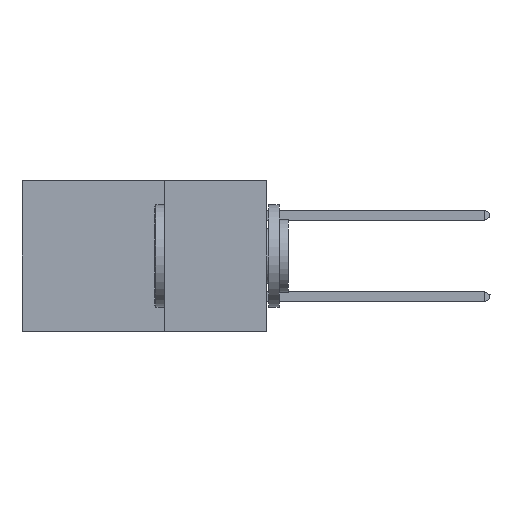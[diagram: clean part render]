
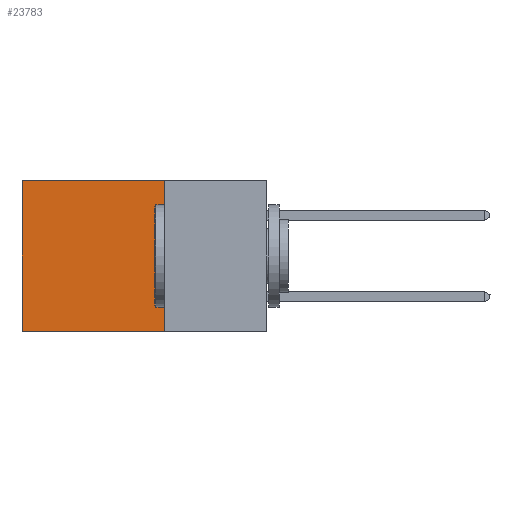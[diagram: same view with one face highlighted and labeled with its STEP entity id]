
A CAD part, left-side view. The second image highlights one B-rep face of the part: STEP entity #23783.
In plain terms, the highlighted planar face has unit normal (-1, 0, 0).
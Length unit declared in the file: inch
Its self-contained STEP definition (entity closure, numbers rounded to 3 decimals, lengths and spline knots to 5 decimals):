
#1271 = CARTESIAN_POINT ( 'NONE',  ( 0.2875, 0.6, -0.37 ) ) ;
#2696 = LINE ( 'NONE', #6786, #36208 ) ;
#3271 = CARTESIAN_POINT ( 'NONE',  ( 0.2875, 0.25, 0. ) ) ;
#5519 = VECTOR ( 'NONE', #27564, 39.37008 ) ;
#5721 = VERTEX_POINT ( 'NONE', #1271 ) ;
#6676 = EDGE_CURVE ( 'NONE', #11344, #39851, #2696, .T. ) ;
#6786 = CARTESIAN_POINT ( 'NONE',  ( 0.2875, 0.25, 0. ) ) ;
#6820 = VERTEX_POINT ( 'NONE', #20052 ) ;
#7052 = LINE ( 'NONE', #31118, #30975 ) ;
#9283 = ORIENTED_EDGE ( 'NONE', *, *, #25885, .F. ) ;
#10921 = ORIENTED_EDGE ( 'NONE', *, *, #6676, .T. ) ;
#11344 = VERTEX_POINT ( 'NONE', #3271 ) ;
#11499 = AXIS2_PLACEMENT_3D ( 'NONE', #22171, #29026, #25544 ) ;
#12484 = ORIENTED_EDGE ( 'NONE', *, *, #43622, .T. ) ;
#17196 = EDGE_LOOP ( 'NONE', ( #12484, #18964, #9283, #10921 ) ) ;
#17632 = CARTESIAN_POINT ( 'NONE',  ( 0.2875, 0.25, -0.37 ) ) ;
#18640 = CARTESIAN_POINT ( 'NONE',  ( 0.2875, 0.25, 0. ) ) ;
#18964 = ORIENTED_EDGE ( 'NONE', *, *, #24275, .F. ) ;
#19941 = FACE_OUTER_BOUND ( 'NONE', #17196, .T. ) ;
#20052 = CARTESIAN_POINT ( 'NONE',  ( 0.2875, 0.25, -0.37 ) ) ;
#20059 = DIRECTION ( 'NONE',  ( 0., 1., 0. ) ) ;
#22063 = DIRECTION ( 'NONE',  ( 0., 0., -1. ) ) ;
#22171 = CARTESIAN_POINT ( 'NONE',  ( 0.2875, 0.25, 0. ) ) ;
#23783 = ADVANCED_FACE ( 'NONE', ( #19941 ), #39420, .F. ) ;
#24275 = EDGE_CURVE ( 'NONE', #6820, #5721, #41738, .T. ) ;
#25544 = DIRECTION ( 'NONE',  ( 0., 0., -1. ) ) ;
#25801 = CARTESIAN_POINT ( 'NONE',  ( 0.2875, 0.6, 0. ) ) ;
#25885 = EDGE_CURVE ( 'NONE', #11344, #6820, #31896, .T. ) ;
#27564 = DIRECTION ( 'NONE',  ( 0., 1., 0. ) ) ;
#29026 = DIRECTION ( 'NONE',  ( 1., 0., 0. ) ) ;
#30975 = VECTOR ( 'NONE', #41101, 39.37008 ) ;
#31118 = CARTESIAN_POINT ( 'NONE',  ( 0.2875, 0.6, 0. ) ) ;
#31896 = LINE ( 'NONE', #18640, #40476 ) ;
#36208 = VECTOR ( 'NONE', #20059, 39.37008 ) ;
#39420 = PLANE ( 'NONE',  #11499 ) ;
#39851 = VERTEX_POINT ( 'NONE', #25801 ) ;
#40476 = VECTOR ( 'NONE', #22063, 39.37008 ) ;
#41101 = DIRECTION ( 'NONE',  ( 0., 0., -1. ) ) ;
#41738 = LINE ( 'NONE', #17632, #5519 ) ;
#43622 = EDGE_CURVE ( 'NONE', #39851, #5721, #7052, .T. ) ;
